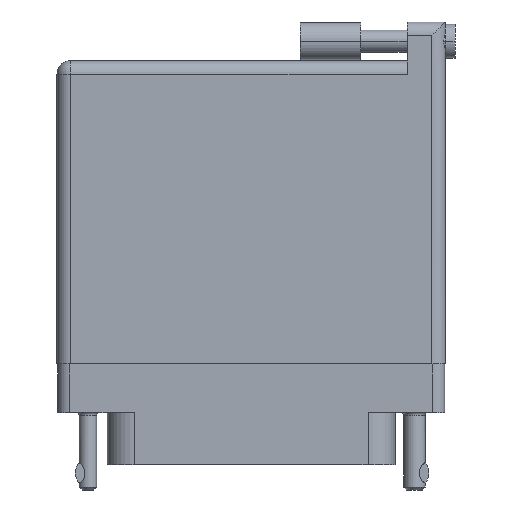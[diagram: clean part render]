
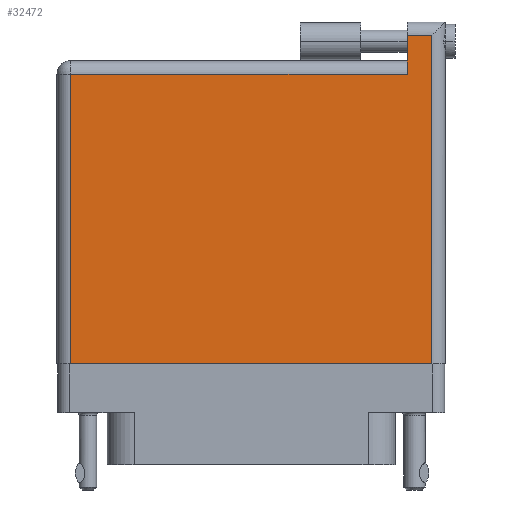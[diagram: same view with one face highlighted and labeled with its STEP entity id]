
A CAD part, front view. The second image highlights one B-rep face of the part: STEP entity #32472.
In plain terms, the highlighted face is planar.
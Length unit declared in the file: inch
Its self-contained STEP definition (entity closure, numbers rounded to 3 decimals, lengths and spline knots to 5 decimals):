
#1682 = CARTESIAN_POINT ( 'NONE',  ( -1.004, 1.596, 0.4495 ) ) ;
#1876 = VECTOR ( 'NONE', #35598, 39.37008 ) ;
#2640 = DIRECTION ( 'NONE',  ( 1., 0., 0. ) ) ;
#3305 = EDGE_CURVE ( 'NONE', #30432, #25913, #19567, .T. ) ;
#5156 = CARTESIAN_POINT ( 'NONE',  ( 0.807, 1.396, 0.4495 ) ) ;
#5397 = CARTESIAN_POINT ( 'NONE',  ( -0.934, -0.1, 0.4495 ) ) ;
#6972 = DIRECTION ( 'NONE',  ( 0., -1., 0. ) ) ;
#7017 = LINE ( 'NONE', #40493, #49071 ) ;
#7459 = ORIENTED_EDGE ( 'NONE', *, *, #40189, .T. ) ;
#8268 = CARTESIAN_POINT ( 'NONE',  ( -0.934, -0.1, 0.4495 ) ) ;
#8762 = LINE ( 'NONE', #18364, #25904 ) ;
#8840 = ORIENTED_EDGE ( 'NONE', *, *, #3305, .T. ) ;
#9005 = FACE_OUTER_BOUND ( 'NONE', #46996, .T. ) ;
#9306 = LINE ( 'NONE', #1682, #29995 ) ;
#10996 = CARTESIAN_POINT ( 'NONE',  ( 0.934, 1.666, 0.4495 ) ) ;
#11154 = DIRECTION ( 'NONE',  ( 0., 1., 0. ) ) ;
#12739 = VERTEX_POINT ( 'NONE', #5397 ) ;
#15468 = VERTEX_POINT ( 'NONE', #40363 ) ;
#18364 = CARTESIAN_POINT ( 'NONE',  ( 0.807, 1.666, 0.4495 ) ) ;
#18370 = DIRECTION ( 'NONE',  ( 0., 0., -1. ) ) ;
#18459 = ORIENTED_EDGE ( 'NONE', *, *, #23465, .T. ) ;
#19495 = DIRECTION ( 'NONE',  ( 0., -1., 0. ) ) ;
#19567 = LINE ( 'NONE', #35092, #1876 ) ;
#23465 = EDGE_CURVE ( 'NONE', #15468, #41834, #26846, .T. ) ;
#23494 = ORIENTED_EDGE ( 'NONE', *, *, #47002, .T. ) ;
#24804 = CARTESIAN_POINT ( 'NONE',  ( 0.807, 1.596, 0.4495 ) ) ;
#25904 = VECTOR ( 'NONE', #6972, 39.37008 ) ;
#25913 = VERTEX_POINT ( 'NONE', #46877 ) ;
#26112 = PLANE ( 'NONE',  #35225 ) ;
#26619 = CARTESIAN_POINT ( 'NONE',  ( -1.004, 1.466, 0.4495 ) ) ;
#26846 = LINE ( 'NONE', #10996, #35774 ) ;
#28307 = EDGE_CURVE ( 'NONE', #40630, #30432, #8762, .T. ) ;
#29782 = ORIENTED_EDGE ( 'NONE', *, *, #40471, .T. ) ;
#29995 = VECTOR ( 'NONE', #47803, 39.37008 ) ;
#30303 = DIRECTION ( 'NONE',  ( -1., 0., 0. ) ) ;
#30432 = VERTEX_POINT ( 'NONE', #5156 ) ;
#32472 = ADVANCED_FACE ( 'NONE', ( #9005 ), #26112, .F. ) ;
#34720 = LINE ( 'NONE', #8268, #46551 ) ;
#35092 = CARTESIAN_POINT ( 'NONE',  ( -1.004, 1.396, 0.4495 ) ) ;
#35225 = AXIS2_PLACEMENT_3D ( 'NONE', #26619, #18370, #30303 ) ;
#35598 = DIRECTION ( 'NONE',  ( -1., 0., 0. ) ) ;
#35774 = VECTOR ( 'NONE', #11154, 39.37008 ) ;
#40189 = EDGE_CURVE ( 'NONE', #41834, #40630, #9306, .T. ) ;
#40343 = CARTESIAN_POINT ( 'NONE',  ( 0.934, 1.596, 0.4495 ) ) ;
#40363 = CARTESIAN_POINT ( 'NONE',  ( 0.934, -0.1, 0.4495 ) ) ;
#40471 = EDGE_CURVE ( 'NONE', #25913, #12739, #34720, .T. ) ;
#40493 = CARTESIAN_POINT ( 'NONE',  ( -1.004, -0.1, 0.4495 ) ) ;
#40630 = VERTEX_POINT ( 'NONE', #24804 ) ;
#41834 = VERTEX_POINT ( 'NONE', #40343 ) ;
#45844 = ORIENTED_EDGE ( 'NONE', *, *, #28307, .T. ) ;
#46551 = VECTOR ( 'NONE', #19495, 39.37008 ) ;
#46877 = CARTESIAN_POINT ( 'NONE',  ( -0.934, 1.396, 0.4495 ) ) ;
#46996 = EDGE_LOOP ( 'NONE', ( #23494, #18459, #7459, #45844, #8840, #29782 ) ) ;
#47002 = EDGE_CURVE ( 'NONE', #12739, #15468, #7017, .T. ) ;
#47803 = DIRECTION ( 'NONE',  ( -1., 0., 0. ) ) ;
#49071 = VECTOR ( 'NONE', #2640, 39.37008 ) ;
